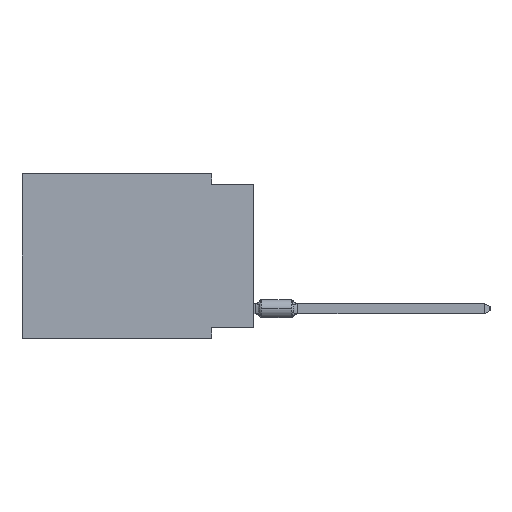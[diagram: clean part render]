
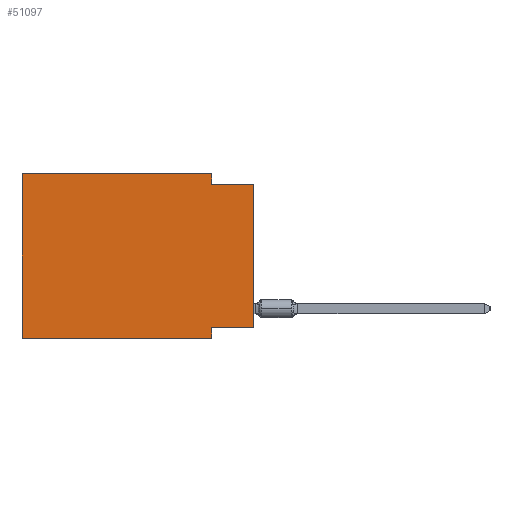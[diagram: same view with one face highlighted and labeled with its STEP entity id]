
A CAD part, left-side view. The second image highlights one B-rep face of the part: STEP entity #51097.
In plain terms, the highlighted planar face has unit normal (-1, 0, 0).
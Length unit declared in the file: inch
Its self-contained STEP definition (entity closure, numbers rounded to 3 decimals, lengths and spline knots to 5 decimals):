
#731 = LINE ( 'NONE', #70193, #43034 ) ;
#2536 = LINE ( 'NONE', #30065, #62034 ) ;
#3309 = VECTOR ( 'NONE', #5361, 39.37008 ) ;
#3681 = DIRECTION ( 'NONE',  ( 0., -1., 0. ) ) ;
#4709 = ORIENTED_EDGE ( 'NONE', *, *, #40102, .F. ) ;
#5361 = DIRECTION ( 'NONE',  ( 0., 0., 1. ) ) ;
#8198 = DIRECTION ( 'NONE',  ( 1., 0., 0. ) ) ;
#8856 = VERTEX_POINT ( 'NONE', #37245 ) ;
#10245 = EDGE_CURVE ( 'NONE', #29203, #8856, #731, .T. ) ;
#10250 = CARTESIAN_POINT ( 'NONE',  ( 0., 0., -0.025 ) ) ;
#10768 = LINE ( 'NONE', #55075, #3309 ) ;
#18448 = CARTESIAN_POINT ( 'NONE',  ( 0., 0.55, 0. ) ) ;
#19423 = CARTESIAN_POINT ( 'NONE',  ( 0., 0.55, 0. ) ) ;
#19520 = DIRECTION ( 'NONE',  ( 0., -1., 0. ) ) ;
#20591 = ORIENTED_EDGE ( 'NONE', *, *, #58467, .T. ) ;
#20857 = VECTOR ( 'NONE', #35163, 39.37008 ) ;
#22630 = VERTEX_POINT ( 'NONE', #65654 ) ;
#24648 = CARTESIAN_POINT ( 'NONE',  ( 0., 0., -0.365 ) ) ;
#25483 = EDGE_CURVE ( 'NONE', #70095, #31188, #32798, .T. ) ;
#27567 = CARTESIAN_POINT ( 'NONE',  ( 0., 0.1, 0. ) ) ;
#27614 = ORIENTED_EDGE ( 'NONE', *, *, #42534, .F. ) ;
#27785 = CARTESIAN_POINT ( 'NONE',  ( 0., 0., -0.365 ) ) ;
#28014 = EDGE_CURVE ( 'NONE', #54473, #52084, #41270, .T. ) ;
#29203 = VERTEX_POINT ( 'NONE', #40221 ) ;
#29309 = DIRECTION ( 'NONE',  ( 0., 0., -1. ) ) ;
#29971 = ORIENTED_EDGE ( 'NONE', *, *, #28014, .F. ) ;
#29990 = VECTOR ( 'NONE', #3681, 39.37008 ) ;
#30065 = CARTESIAN_POINT ( 'NONE',  ( 0., 0.55, -0.39 ) ) ;
#31153 = DIRECTION ( 'NONE',  ( 0., 1., 0. ) ) ;
#31188 = VERTEX_POINT ( 'NONE', #10250 ) ;
#32798 = LINE ( 'NONE', #44056, #34839 ) ;
#34839 = VECTOR ( 'NONE', #55319, 39.37008 ) ;
#35163 = DIRECTION ( 'NONE',  ( 0., -1., 0. ) ) ;
#37245 = CARTESIAN_POINT ( 'NONE',  ( 0., 0.1, -0.39 ) ) ;
#38369 = CARTESIAN_POINT ( 'NONE',  ( 0., 0.1, -0.025 ) ) ;
#38902 = CARTESIAN_POINT ( 'NONE',  ( 0., 0.55, 0. ) ) ;
#40102 = EDGE_CURVE ( 'NONE', #70095, #29203, #43753, .T. ) ;
#40221 = CARTESIAN_POINT ( 'NONE',  ( 0., 0.1, -0.365 ) ) ;
#41270 = LINE ( 'NONE', #68456, #42666 ) ;
#41469 = ORIENTED_EDGE ( 'NONE', *, *, #10245, .F. ) ;
#42390 = VECTOR ( 'NONE', #31153, 39.37008 ) ;
#42534 = EDGE_CURVE ( 'NONE', #63342, #54473, #69573, .T. ) ;
#42666 = VECTOR ( 'NONE', #29309, 39.37008 ) ;
#43034 = VECTOR ( 'NONE', #67796, 39.37008 ) ;
#43753 = LINE ( 'NONE', #24648, #42390 ) ;
#44056 = CARTESIAN_POINT ( 'NONE',  ( 0., 0., 0. ) ) ;
#44712 = AXIS2_PLACEMENT_3D ( 'NONE', #19423, #8198, #69853 ) ;
#45789 = ORIENTED_EDGE ( 'NONE', *, *, #63612, .F. ) ;
#47354 = EDGE_LOOP ( 'NONE', ( #59702, #66591, #29971, #27614, #45789, #20591, #41469, #4709 ) ) ;
#51097 = ADVANCED_FACE ( 'NONE', ( #52840 ), #58272, .F. ) ;
#51943 = CARTESIAN_POINT ( 'NONE',  ( 0., 0., -0.025 ) ) ;
#52084 = VERTEX_POINT ( 'NONE', #38369 ) ;
#52840 = FACE_OUTER_BOUND ( 'NONE', #47354, .T. ) ;
#54473 = VERTEX_POINT ( 'NONE', #27567 ) ;
#55075 = CARTESIAN_POINT ( 'NONE',  ( 0., 0.55, 0. ) ) ;
#55319 = DIRECTION ( 'NONE',  ( 0., 0., 1. ) ) ;
#58272 = PLANE ( 'NONE',  #44712 ) ;
#58467 = EDGE_CURVE ( 'NONE', #22630, #8856, #2536, .T. ) ;
#59702 = ORIENTED_EDGE ( 'NONE', *, *, #25483, .T. ) ;
#62034 = VECTOR ( 'NONE', #19520, 39.37008 ) ;
#63342 = VERTEX_POINT ( 'NONE', #38902 ) ;
#63612 = EDGE_CURVE ( 'NONE', #22630, #63342, #10768, .T. ) ;
#64704 = EDGE_CURVE ( 'NONE', #52084, #31188, #68964, .T. ) ;
#65654 = CARTESIAN_POINT ( 'NONE',  ( 0., 0.55, -0.39 ) ) ;
#66591 = ORIENTED_EDGE ( 'NONE', *, *, #64704, .F. ) ;
#67796 = DIRECTION ( 'NONE',  ( 0., 0., -1. ) ) ;
#68456 = CARTESIAN_POINT ( 'NONE',  ( 0., 0.1, 0. ) ) ;
#68964 = LINE ( 'NONE', #51943, #29990 ) ;
#69573 = LINE ( 'NONE', #18448, #20857 ) ;
#69853 = DIRECTION ( 'NONE',  ( 0., 0., -1. ) ) ;
#70095 = VERTEX_POINT ( 'NONE', #27785 ) ;
#70193 = CARTESIAN_POINT ( 'NONE',  ( 0., 0.1, -0.39 ) ) ;
